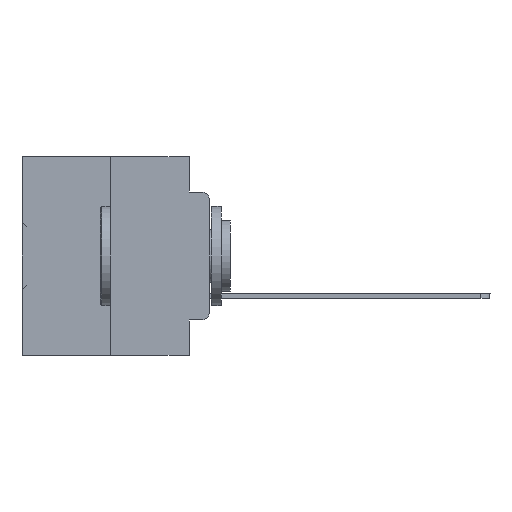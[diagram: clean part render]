
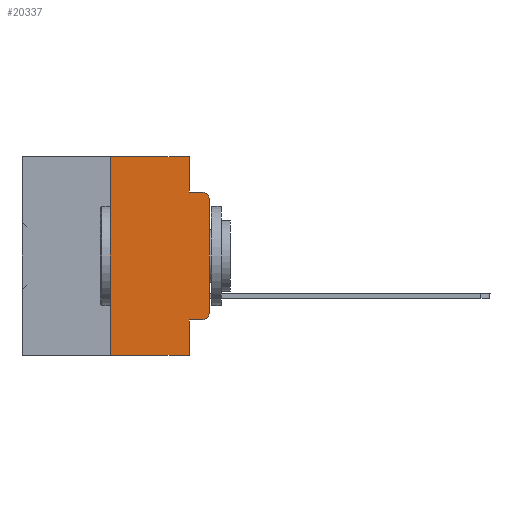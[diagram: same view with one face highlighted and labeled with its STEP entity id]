
A CAD part, left-side view. The second image highlights one B-rep face of the part: STEP entity #20337.
In plain terms, the highlighted planar face has unit normal (-1, 0, 0).
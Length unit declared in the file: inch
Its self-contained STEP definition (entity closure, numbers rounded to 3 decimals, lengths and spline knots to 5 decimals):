
#57 = EDGE_CURVE ( 'NONE', #10081, #23240, #29617, .T. ) ;
#486 = DIRECTION ( 'NONE',  ( 0., 0., -1. ) ) ;
#859 = CARTESIAN_POINT ( 'NONE',  ( 0., 0.473, 0. ) ) ;
#1043 = EDGE_LOOP ( 'NONE', ( #14530, #17052, #11345, #15751, #18547, #29742, #3253, #2582, #25674, #8651 ) ) ;
#2348 = VECTOR ( 'NONE', #9195, 39.37008 ) ;
#2582 = ORIENTED_EDGE ( 'NONE', *, *, #36299, .F. ) ;
#2824 = AXIS2_PLACEMENT_3D ( 'NONE', #859, #6792, #15187 ) ;
#2888 = CARTESIAN_POINT ( 'NONE',  ( 0., 0.051, -0.4115 ) ) ;
#2975 = DIRECTION ( 'NONE',  ( -1., 0., 0. ) ) ;
#3132 = CARTESIAN_POINT ( 'NONE',  ( 0., 0.051, 0. ) ) ;
#3163 = PLANE ( 'NONE',  #2824 ) ;
#3253 = ORIENTED_EDGE ( 'NONE', *, *, #29053, .T. ) ;
#3672 = CARTESIAN_POINT ( 'NONE',  ( 0., 0.051, 0. ) ) ;
#4378 = AXIS2_PLACEMENT_3D ( 'NONE', #11831, #35135, #36420 ) ;
#4775 = DIRECTION ( 'NONE',  ( 0., 0., 1. ) ) ;
#5577 = CIRCLE ( 'NONE', #4378, 0.02 ) ;
#5891 = EDGE_CURVE ( 'NONE', #23240, #23340, #29840, .T. ) ;
#6132 = CARTESIAN_POINT ( 'NONE',  ( 0., 0.473, -0.5 ) ) ;
#6388 = CARTESIAN_POINT ( 'NONE',  ( 0., 0.051, -0.0885 ) ) ;
#6792 = DIRECTION ( 'NONE',  ( 1., 0., 0. ) ) ;
#7287 = LINE ( 'NONE', #27722, #17019 ) ;
#8042 = LINE ( 'NONE', #16263, #31044 ) ;
#8313 = VERTEX_POINT ( 'NONE', #28407 ) ;
#8651 = ORIENTED_EDGE ( 'NONE', *, *, #31932, .T. ) ;
#8882 = VECTOR ( 'NONE', #21264, 39.37008 ) ;
#9195 = DIRECTION ( 'NONE',  ( 0., -1., 0. ) ) ;
#9285 = CARTESIAN_POINT ( 'NONE',  ( 0., 0.02, -0.3915 ) ) ;
#9615 = LINE ( 'NONE', #32899, #8882 ) ;
#9660 = FACE_OUTER_BOUND ( 'NONE', #1043, .T. ) ;
#10081 = VERTEX_POINT ( 'NONE', #16506 ) ;
#10321 = CARTESIAN_POINT ( 'NONE',  ( 0., 0., -0.3915 ) ) ;
#10494 = VERTEX_POINT ( 'NONE', #10321 ) ;
#11345 = ORIENTED_EDGE ( 'NONE', *, *, #37417, .F. ) ;
#11633 = LINE ( 'NONE', #31687, #25898 ) ;
#11662 = CIRCLE ( 'NONE', #32995, 0.02 ) ;
#11831 = CARTESIAN_POINT ( 'NONE',  ( 0., 0.02, -0.1085 ) ) ;
#12287 = DIRECTION ( 'NONE',  ( 0., 0., -1. ) ) ;
#14530 = ORIENTED_EDGE ( 'NONE', *, *, #36195, .T. ) ;
#15187 = DIRECTION ( 'NONE',  ( 0., 0., -1. ) ) ;
#15282 = CARTESIAN_POINT ( 'NONE',  ( 0., 0.473, 0. ) ) ;
#15751 = ORIENTED_EDGE ( 'NONE', *, *, #5891, .F. ) ;
#16263 = CARTESIAN_POINT ( 'NONE',  ( 0., 0.25, 0. ) ) ;
#16506 = CARTESIAN_POINT ( 'NONE',  ( 0., 0.25, 0. ) ) ;
#16608 = DIRECTION ( 'NONE',  ( 0., 0., -1. ) ) ;
#16728 = VECTOR ( 'NONE', #4775, 39.37008 ) ;
#16844 = VERTEX_POINT ( 'NONE', #37489 ) ;
#17019 = VECTOR ( 'NONE', #22380, 39.37008 ) ;
#17052 = ORIENTED_EDGE ( 'NONE', *, *, #33449, .T. ) ;
#17554 = VERTEX_POINT ( 'NONE', #36786 ) ;
#17789 = LINE ( 'NONE', #6132, #2348 ) ;
#18547 = ORIENTED_EDGE ( 'NONE', *, *, #57, .F. ) ;
#20053 = CARTESIAN_POINT ( 'NONE',  ( 0., 0.25, -0.5 ) ) ;
#20337 = ADVANCED_FACE ( 'NONE', ( #9660 ), #3163, .F. ) ;
#20836 = DIRECTION ( 'NONE',  ( 0., -1., 0. ) ) ;
#21017 = VERTEX_POINT ( 'NONE', #20053 ) ;
#21264 = DIRECTION ( 'NONE',  ( 0., -1., 0. ) ) ;
#22380 = DIRECTION ( 'NONE',  ( 0., -1., 0. ) ) ;
#23240 = VERTEX_POINT ( 'NONE', #3132 ) ;
#23340 = VERTEX_POINT ( 'NONE', #6388 ) ;
#25105 = EDGE_CURVE ( 'NONE', #27745, #8313, #7287, .T. ) ;
#25218 = CARTESIAN_POINT ( 'NONE',  ( 0., 0., 0. ) ) ;
#25603 = DIRECTION ( 'NONE',  ( 0., 0., 1. ) ) ;
#25674 = ORIENTED_EDGE ( 'NONE', *, *, #25105, .T. ) ;
#25898 = VECTOR ( 'NONE', #16608, 39.37008 ) ;
#26391 = CARTESIAN_POINT ( 'NONE',  ( 0., 0., -0.1085 ) ) ;
#27511 = LINE ( 'NONE', #25218, #16728 ) ;
#27722 = CARTESIAN_POINT ( 'NONE',  ( 0., 0.051, -0.4115 ) ) ;
#27726 = VERTEX_POINT ( 'NONE', #26391 ) ;
#27745 = VERTEX_POINT ( 'NONE', #2888 ) ;
#28407 = CARTESIAN_POINT ( 'NONE',  ( 0., 0.02, -0.4115 ) ) ;
#28679 = VECTOR ( 'NONE', #20836, 39.37008 ) ;
#29053 = EDGE_CURVE ( 'NONE', #21017, #17554, #17789, .T. ) ;
#29334 = EDGE_CURVE ( 'NONE', #21017, #10081, #8042, .T. ) ;
#29617 = LINE ( 'NONE', #15282, #28679 ) ;
#29742 = ORIENTED_EDGE ( 'NONE', *, *, #29334, .F. ) ;
#29840 = LINE ( 'NONE', #3672, #30008 ) ;
#30008 = VECTOR ( 'NONE', #12287, 39.37008 ) ;
#31044 = VECTOR ( 'NONE', #25603, 39.37008 ) ;
#31687 = CARTESIAN_POINT ( 'NONE',  ( 0., 0.051, 0. ) ) ;
#31932 = EDGE_CURVE ( 'NONE', #8313, #10494, #11662, .T. ) ;
#32899 = CARTESIAN_POINT ( 'NONE',  ( 0., 0.051, -0.0885 ) ) ;
#32995 = AXIS2_PLACEMENT_3D ( 'NONE', #9285, #2975, #486 ) ;
#33449 = EDGE_CURVE ( 'NONE', #27726, #16844, #5577, .T. ) ;
#35135 = DIRECTION ( 'NONE',  ( -1., 0., 0. ) ) ;
#36195 = EDGE_CURVE ( 'NONE', #10494, #27726, #27511, .T. ) ;
#36299 = EDGE_CURVE ( 'NONE', #27745, #17554, #11633, .T. ) ;
#36420 = DIRECTION ( 'NONE',  ( 0., 0., -1. ) ) ;
#36786 = CARTESIAN_POINT ( 'NONE',  ( 0., 0.051, -0.5 ) ) ;
#37417 = EDGE_CURVE ( 'NONE', #23340, #16844, #9615, .T. ) ;
#37489 = CARTESIAN_POINT ( 'NONE',  ( 0., 0.02, -0.0885 ) ) ;
